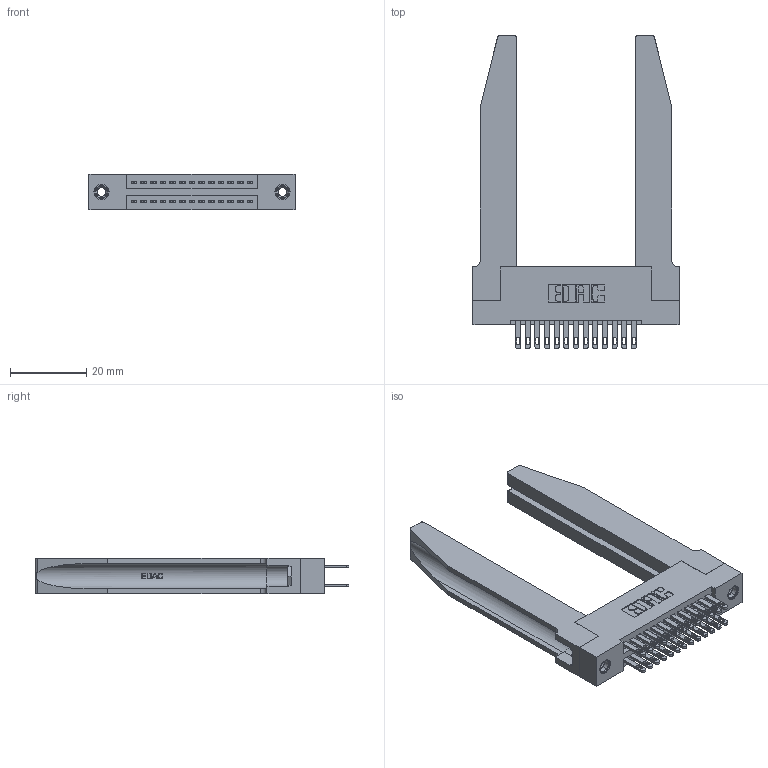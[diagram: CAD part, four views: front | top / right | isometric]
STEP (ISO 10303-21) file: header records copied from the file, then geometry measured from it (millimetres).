
FILE_DESCRIPTION (( 'STEP AP203' ), '1' );
FILE_NAME ('345-026-500-278.STEP', '2019-10-27T18:18:17', ( '' ), ( '' ), 'SwSTEP 2.0', 'SolidWorks 2016', '' );
FILE_SCHEMA (( 'CONFIG_CONTROL_DESIGN' ));
Length unit declared in the file: inch
Products named in the file (5): 345-250-001_345-250-001-102; 345-026-500-278; 345 Part_Flush Mounting Lugs - 0.156 Dia-TH; 345-220-078_345-220-078; 345-292-001_345-293-100
Assembly tree (31 placements, depth 2):
  345-026-500-278
    345 Part_Flush Mounting Lugs - 0.156 Dia-TH
    345-292-001_345-293-100  x26
    345-250-001_345-250-001-102  x2
    345-220-078_345-220-078  x2
Bounding box: 54.25 x 82.47 x 9.4 mm (x, y, z)
Volume: 12851 mm3; surface area: 14051.9 mm2
Topology: 31 solids, 31 shells, 1556 faces, 4615 edges, 3066 vertices
Faces by surface type: plane 924, cylinder 580, bspline 36, cone 12, torus 4
Entity records: 18774 total; most frequent: CARTESIAN_POINT 4091, ORIENTED_EDGE 2922, DIRECTION 2639, EDGE_CURVE 1461, VECTOR 1179, LINE 1179, VERTEX_POINT 968, AXIS2_PLACEMENT_3D 730
